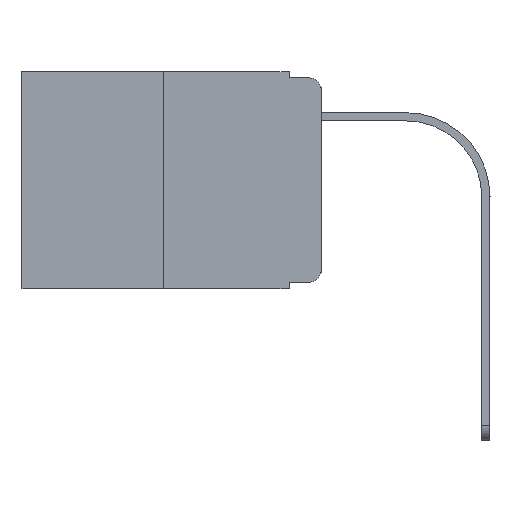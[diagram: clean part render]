
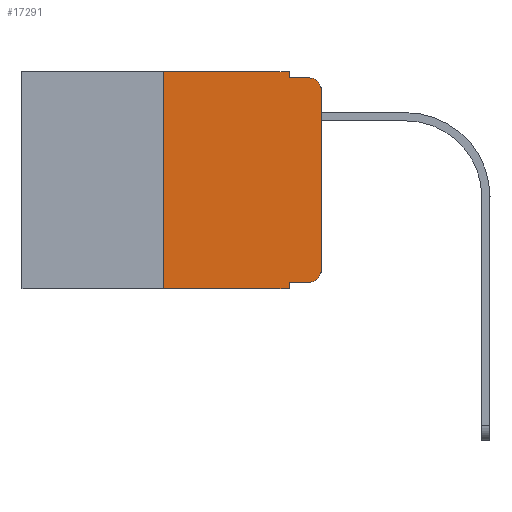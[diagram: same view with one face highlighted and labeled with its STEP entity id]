
A CAD part, left-side view. The second image highlights one B-rep face of the part: STEP entity #17291.
In plain terms, the highlighted planar face has unit normal (-1, 0, 0).
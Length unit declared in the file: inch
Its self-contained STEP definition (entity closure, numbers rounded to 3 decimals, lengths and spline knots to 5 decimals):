
#434 = LINE ( 'NONE', #13133, #9205 ) ;
#489 = LINE ( 'NONE', #14582, #5699 ) ;
#1169 = DIRECTION ( 'NONE',  ( 0., -1., 0. ) ) ;
#1342 = CARTESIAN_POINT ( 'NONE',  ( 0., 0.02, -0.01 ) ) ;
#1348 = AXIS2_PLACEMENT_3D ( 'NONE', #8318, #2696, #5570 ) ;
#1557 = ORIENTED_EDGE ( 'NONE', *, *, #2551, .F. ) ;
#1894 = EDGE_CURVE ( 'NONE', #17871, #7409, #7406, .T. ) ;
#1910 = DIRECTION ( 'NONE',  ( 0., 0., 1. ) ) ;
#1999 = ORIENTED_EDGE ( 'NONE', *, *, #16993, .T. ) ;
#2238 = CARTESIAN_POINT ( 'NONE',  ( 0., 0., -0.313 ) ) ;
#2551 = EDGE_CURVE ( 'NONE', #8747, #9998, #9644, .T. ) ;
#2696 = DIRECTION ( 'NONE',  ( 1., 0., 0. ) ) ;
#2729 = EDGE_CURVE ( 'NONE', #12361, #8747, #7153, .T. ) ;
#2830 = CARTESIAN_POINT ( 'NONE',  ( 0., 0.051, 0. ) ) ;
#3095 = DIRECTION ( 'NONE',  ( 0., 0., 1. ) ) ;
#3119 = ORIENTED_EDGE ( 'NONE', *, *, #10419, .F. ) ;
#3261 = CARTESIAN_POINT ( 'NONE',  ( 0., 0.473, 0. ) ) ;
#3525 = CARTESIAN_POINT ( 'NONE',  ( 0., 0.02, -0.313 ) ) ;
#3622 = DIRECTION ( 'NONE',  ( -1., 0., 0. ) ) ;
#3721 = DIRECTION ( 'NONE',  ( 0., 0., -1. ) ) ;
#4396 = DIRECTION ( 'NONE',  ( 0., 0., -1. ) ) ;
#4885 = CARTESIAN_POINT ( 'NONE',  ( 0., 0.051, 0. ) ) ;
#5005 = VECTOR ( 'NONE', #12679, 39.37008 ) ;
#5262 = EDGE_LOOP ( 'NONE', ( #1999, #6207, #1557, #18036, #12764, #3119, #12928, #13370, #16298, #13417 ) ) ;
#5403 = AXIS2_PLACEMENT_3D ( 'NONE', #9727, #17004, #4396 ) ;
#5570 = DIRECTION ( 'NONE',  ( 0., 0., -1. ) ) ;
#5697 = EDGE_CURVE ( 'NONE', #6547, #17871, #434, .T. ) ;
#5699 = VECTOR ( 'NONE', #11523, 39.37008 ) ;
#5742 = EDGE_CURVE ( 'NONE', #9151, #12361, #8985, .T. ) ;
#6207 = ORIENTED_EDGE ( 'NONE', *, *, #10322, .T. ) ;
#6269 = CIRCLE ( 'NONE', #5403, 0.02 ) ;
#6323 = CARTESIAN_POINT ( 'NONE',  ( 0., 0.25, 0. ) ) ;
#6493 = CARTESIAN_POINT ( 'NONE',  ( 0., 0.051, -0.343 ) ) ;
#6547 = VERTEX_POINT ( 'NONE', #9918 ) ;
#7052 = VECTOR ( 'NONE', #1169, 39.37008 ) ;
#7153 = LINE ( 'NONE', #2830, #5005 ) ;
#7378 = VECTOR ( 'NONE', #10489, 39.37008 ) ;
#7406 = CIRCLE ( 'NONE', #16232, 0.02 ) ;
#7409 = VERTEX_POINT ( 'NONE', #2238 ) ;
#7635 = EDGE_CURVE ( 'NONE', #17700, #9885, #489, .T. ) ;
#8028 = VECTOR ( 'NONE', #15892, 39.37008 ) ;
#8282 = EDGE_CURVE ( 'NONE', #6547, #9885, #17472, .T. ) ;
#8318 = CARTESIAN_POINT ( 'NONE',  ( 0., 0.473, 0. ) ) ;
#8417 = FACE_OUTER_BOUND ( 'NONE', #5262, .T. ) ;
#8747 = VERTEX_POINT ( 'NONE', #17039 ) ;
#8985 = LINE ( 'NONE', #3261, #8028 ) ;
#9151 = VERTEX_POINT ( 'NONE', #17873 ) ;
#9205 = VECTOR ( 'NONE', #15981, 39.37008 ) ;
#9644 = LINE ( 'NONE', #12146, #7052 ) ;
#9727 = CARTESIAN_POINT ( 'NONE',  ( 0., 0.02, -0.03 ) ) ;
#9809 = CARTESIAN_POINT ( 'NONE',  ( 0., 0., -0.03 ) ) ;
#9885 = VERTEX_POINT ( 'NONE', #6493 ) ;
#9918 = CARTESIAN_POINT ( 'NONE',  ( 0., 0.051, -0.333 ) ) ;
#9998 = VERTEX_POINT ( 'NONE', #1342 ) ;
#10322 = EDGE_CURVE ( 'NONE', #11998, #9998, #6269, .T. ) ;
#10419 = EDGE_CURVE ( 'NONE', #17700, #9151, #10548, .T. ) ;
#10489 = DIRECTION ( 'NONE',  ( 0., 0., -1. ) ) ;
#10548 = LINE ( 'NONE', #6323, #12170 ) ;
#10907 = PLANE ( 'NONE',  #1348 ) ;
#11523 = DIRECTION ( 'NONE',  ( 0., -1., 0. ) ) ;
#11770 = CARTESIAN_POINT ( 'NONE',  ( 0., 0.02, -0.333 ) ) ;
#11998 = VERTEX_POINT ( 'NONE', #9809 ) ;
#12146 = CARTESIAN_POINT ( 'NONE',  ( 0., 0.051, -0.01 ) ) ;
#12170 = VECTOR ( 'NONE', #1910, 39.37008 ) ;
#12361 = VERTEX_POINT ( 'NONE', #15693 ) ;
#12679 = DIRECTION ( 'NONE',  ( 0., 0., -1. ) ) ;
#12764 = ORIENTED_EDGE ( 'NONE', *, *, #5742, .F. ) ;
#12928 = ORIENTED_EDGE ( 'NONE', *, *, #7635, .T. ) ;
#13133 = CARTESIAN_POINT ( 'NONE',  ( 0., 0.051, -0.333 ) ) ;
#13370 = ORIENTED_EDGE ( 'NONE', *, *, #8282, .F. ) ;
#13417 = ORIENTED_EDGE ( 'NONE', *, *, #1894, .T. ) ;
#13686 = VECTOR ( 'NONE', #3095, 39.37008 ) ;
#14351 = LINE ( 'NONE', #15812, #13686 ) ;
#14582 = CARTESIAN_POINT ( 'NONE',  ( 0., 0.473, -0.343 ) ) ;
#15209 = CARTESIAN_POINT ( 'NONE',  ( 0., 0.25, -0.343 ) ) ;
#15693 = CARTESIAN_POINT ( 'NONE',  ( 0., 0.051, 0. ) ) ;
#15812 = CARTESIAN_POINT ( 'NONE',  ( 0., 0., 0. ) ) ;
#15892 = DIRECTION ( 'NONE',  ( 0., -1., 0. ) ) ;
#15981 = DIRECTION ( 'NONE',  ( 0., -1., 0. ) ) ;
#16232 = AXIS2_PLACEMENT_3D ( 'NONE', #3525, #3622, #3721 ) ;
#16298 = ORIENTED_EDGE ( 'NONE', *, *, #5697, .T. ) ;
#16993 = EDGE_CURVE ( 'NONE', #7409, #11998, #14351, .T. ) ;
#17004 = DIRECTION ( 'NONE',  ( -1., 0., 0. ) ) ;
#17039 = CARTESIAN_POINT ( 'NONE',  ( 0., 0.051, -0.01 ) ) ;
#17291 = ADVANCED_FACE ( 'NONE', ( #8417 ), #10907, .F. ) ;
#17472 = LINE ( 'NONE', #4885, #7378 ) ;
#17700 = VERTEX_POINT ( 'NONE', #15209 ) ;
#17871 = VERTEX_POINT ( 'NONE', #11770 ) ;
#17873 = CARTESIAN_POINT ( 'NONE',  ( 0., 0.25, 0. ) ) ;
#18036 = ORIENTED_EDGE ( 'NONE', *, *, #2729, .F. ) ;
